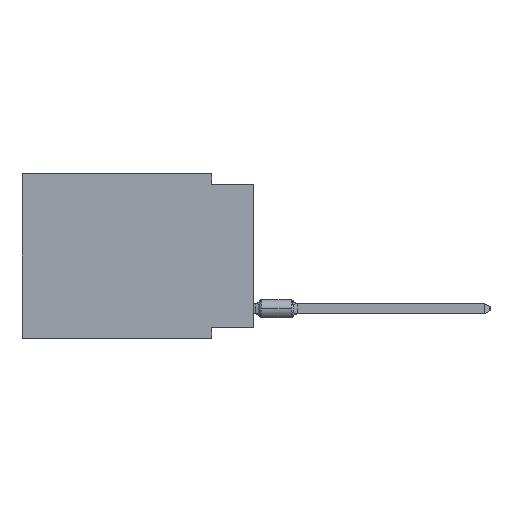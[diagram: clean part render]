
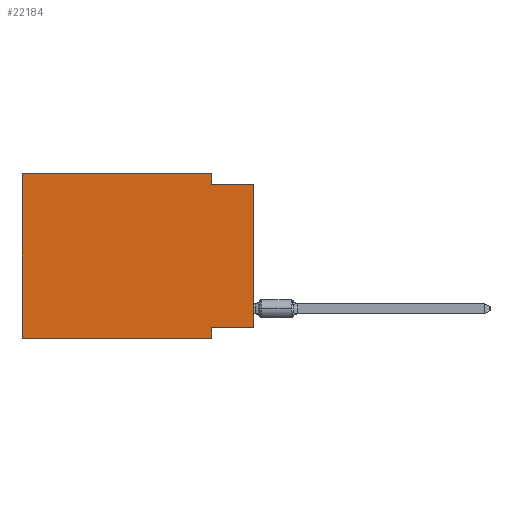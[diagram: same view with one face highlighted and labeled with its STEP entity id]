
A CAD part, left-side view. The second image highlights one B-rep face of the part: STEP entity #22184.
In plain terms, the highlighted planar face has unit normal (-1, 0, 0).
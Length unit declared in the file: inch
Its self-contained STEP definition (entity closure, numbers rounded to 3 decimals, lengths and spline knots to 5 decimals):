
#1909 = AXIS2_PLACEMENT_3D ( 'NONE', #2978, #35117, #27132 ) ;
#1957 = VERTEX_POINT ( 'NONE', #41605 ) ;
#2978 = CARTESIAN_POINT ( 'NONE',  ( 0., 0.55, 0. ) ) ;
#3338 = DIRECTION ( 'NONE',  ( 0., -1., 0. ) ) ;
#4110 = CARTESIAN_POINT ( 'NONE',  ( 0., 0.55, -0.39 ) ) ;
#6626 = EDGE_CURVE ( 'NONE', #34386, #34939, #45149, .T. ) ;
#7210 = LINE ( 'NONE', #15176, #37020 ) ;
#9978 = ORIENTED_EDGE ( 'NONE', *, *, #6626, .F. ) ;
#11132 = VECTOR ( 'NONE', #30987, 39.37008 ) ;
#11204 = PLANE ( 'NONE',  #1909 ) ;
#11458 = ORIENTED_EDGE ( 'NONE', *, *, #14979, .F. ) ;
#12767 = CARTESIAN_POINT ( 'NONE',  ( 0., 0., -0.025 ) ) ;
#13739 = EDGE_CURVE ( 'NONE', #1957, #40353, #51171, .T. ) ;
#14319 = DIRECTION ( 'NONE',  ( 0., 0., 1. ) ) ;
#14979 = EDGE_CURVE ( 'NONE', #18341, #39426, #33606, .T. ) ;
#15176 = CARTESIAN_POINT ( 'NONE',  ( 0., 0., 0. ) ) ;
#15289 = LINE ( 'NONE', #4110, #17983 ) ;
#15320 = ORIENTED_EDGE ( 'NONE', *, *, #28894, .T. ) ;
#16037 = VECTOR ( 'NONE', #41293, 39.37008 ) ;
#17278 = DIRECTION ( 'NONE',  ( 0., 1., 0. ) ) ;
#17983 = VECTOR ( 'NONE', #3338, 39.37008 ) ;
#18341 = VERTEX_POINT ( 'NONE', #25820 ) ;
#19264 = ORIENTED_EDGE ( 'NONE', *, *, #52430, .T. ) ;
#19305 = VERTEX_POINT ( 'NONE', #37054 ) ;
#21008 = CARTESIAN_POINT ( 'NONE',  ( 0., 0., -0.365 ) ) ;
#22184 = ADVANCED_FACE ( 'NONE', ( #34587 ), #11204, .F. ) ;
#25820 = CARTESIAN_POINT ( 'NONE',  ( 0., 0.55, 0. ) ) ;
#27132 = DIRECTION ( 'NONE',  ( 0., 0., -1. ) ) ;
#27199 = VECTOR ( 'NONE', #46356, 39.37008 ) ;
#27993 = ORIENTED_EDGE ( 'NONE', *, *, #13739, .F. ) ;
#28463 = CARTESIAN_POINT ( 'NONE',  ( 0., 0., -0.025 ) ) ;
#28758 = VERTEX_POINT ( 'NONE', #38578 ) ;
#28894 = EDGE_CURVE ( 'NONE', #19305, #34939, #7210, .T. ) ;
#29751 = DIRECTION ( 'NONE',  ( 0., -1., 0. ) ) ;
#30987 = DIRECTION ( 'NONE',  ( 0., 0., -1. ) ) ;
#30993 = EDGE_LOOP ( 'NONE', ( #15320, #9978, #51142, #11458, #42243, #19264, #27993, #51615 ) ) ;
#33606 = LINE ( 'NONE', #45559, #27199 ) ;
#34386 = VERTEX_POINT ( 'NONE', #45623 ) ;
#34562 = CARTESIAN_POINT ( 'NONE',  ( 0., 0.1, -0.39 ) ) ;
#34587 = FACE_OUTER_BOUND ( 'NONE', #30993, .T. ) ;
#34939 = VERTEX_POINT ( 'NONE', #28463 ) ;
#35117 = DIRECTION ( 'NONE',  ( 1., 0., 0. ) ) ;
#37020 = VECTOR ( 'NONE', #52329, 39.37008 ) ;
#37054 = CARTESIAN_POINT ( 'NONE',  ( 0., 0., -0.365 ) ) ;
#38230 = VECTOR ( 'NONE', #17278, 39.37008 ) ;
#38578 = CARTESIAN_POINT ( 'NONE',  ( 0., 0.55, -0.39 ) ) ;
#38831 = VECTOR ( 'NONE', #29751, 39.37008 ) ;
#39426 = VERTEX_POINT ( 'NONE', #52309 ) ;
#40353 = VERTEX_POINT ( 'NONE', #34562 ) ;
#41177 = LINE ( 'NONE', #21008, #38230 ) ;
#41293 = DIRECTION ( 'NONE',  ( 0., 0., -1. ) ) ;
#41552 = LINE ( 'NONE', #45793, #16037 ) ;
#41605 = CARTESIAN_POINT ( 'NONE',  ( 0., 0.1, -0.365 ) ) ;
#42243 = ORIENTED_EDGE ( 'NONE', *, *, #50696, .F. ) ;
#43131 = EDGE_CURVE ( 'NONE', #39426, #34386, #41552, .T. ) ;
#43226 = LINE ( 'NONE', #47475, #45915 ) ;
#44998 = EDGE_CURVE ( 'NONE', #19305, #1957, #41177, .T. ) ;
#45149 = LINE ( 'NONE', #12767, #38831 ) ;
#45559 = CARTESIAN_POINT ( 'NONE',  ( 0., 0.55, 0. ) ) ;
#45623 = CARTESIAN_POINT ( 'NONE',  ( 0., 0.1, -0.025 ) ) ;
#45793 = CARTESIAN_POINT ( 'NONE',  ( 0., 0.1, 0. ) ) ;
#45915 = VECTOR ( 'NONE', #14319, 39.37008 ) ;
#46356 = DIRECTION ( 'NONE',  ( 0., -1., 0. ) ) ;
#47475 = CARTESIAN_POINT ( 'NONE',  ( 0., 0.55, 0. ) ) ;
#50696 = EDGE_CURVE ( 'NONE', #28758, #18341, #43226, .T. ) ;
#51142 = ORIENTED_EDGE ( 'NONE', *, *, #43131, .F. ) ;
#51171 = LINE ( 'NONE', #51414, #11132 ) ;
#51414 = CARTESIAN_POINT ( 'NONE',  ( 0., 0.1, -0.39 ) ) ;
#51615 = ORIENTED_EDGE ( 'NONE', *, *, #44998, .F. ) ;
#52309 = CARTESIAN_POINT ( 'NONE',  ( 0., 0.1, 0. ) ) ;
#52329 = DIRECTION ( 'NONE',  ( 0., 0., 1. ) ) ;
#52430 = EDGE_CURVE ( 'NONE', #28758, #40353, #15289, .T. ) ;
